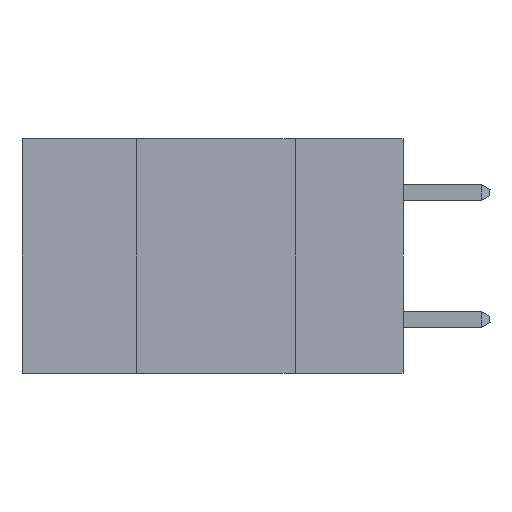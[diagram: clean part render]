
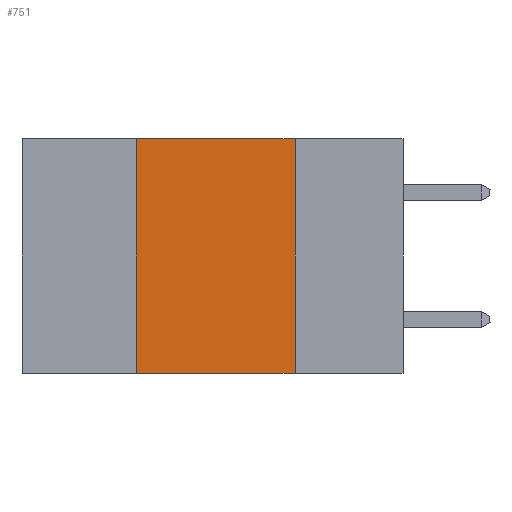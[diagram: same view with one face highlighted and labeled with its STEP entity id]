
A CAD part, left-side view. The second image highlights one B-rep face of the part: STEP entity #751.
In plain terms, the highlighted planar face has unit normal (-1, 0, 0).
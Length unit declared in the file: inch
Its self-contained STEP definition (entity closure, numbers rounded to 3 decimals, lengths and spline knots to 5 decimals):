
#44 = ORIENTED_EDGE ( 'NONE', *, *, #5355, .T. ) ;
#585 = DIRECTION ( 'NONE',  ( 1., 0., 0. ) ) ;
#751 = ADVANCED_FACE ( 'NONE', ( #8405 ), #1571, .F. ) ;
#951 = VERTEX_POINT ( 'NONE', #10991 ) ;
#1030 = AXIS2_PLACEMENT_3D ( 'NONE', #3558, #585, #1523 ) ;
#1355 = CARTESIAN_POINT ( 'NONE',  ( 0., 0.42, 0. ) ) ;
#1523 = DIRECTION ( 'NONE',  ( 0., 0., -1. ) ) ;
#1571 = PLANE ( 'NONE',  #1030 ) ;
#2040 = VECTOR ( 'NONE', #3568, 39.37008 ) ;
#2195 = CARTESIAN_POINT ( 'NONE',  ( 0., 0.17, 0. ) ) ;
#3198 = LINE ( 'NONE', #1355, #9947 ) ;
#3558 = CARTESIAN_POINT ( 'NONE',  ( 0., 0.6, 0. ) ) ;
#3568 = DIRECTION ( 'NONE',  ( 0., -1., 0. ) ) ;
#3680 = CARTESIAN_POINT ( 'NONE',  ( 0., 0.17, 0. ) ) ;
#4013 = LINE ( 'NONE', #2195, #4184 ) ;
#4184 = VECTOR ( 'NONE', #10307, 39.37008 ) ;
#4647 = VERTEX_POINT ( 'NONE', #4947 ) ;
#4910 = CARTESIAN_POINT ( 'NONE',  ( 0., 0.6, 0. ) ) ;
#4947 = CARTESIAN_POINT ( 'NONE',  ( 0., 0.42, -0.37 ) ) ;
#5355 = EDGE_CURVE ( 'NONE', #4647, #7803, #7987, .T. ) ;
#5871 = VECTOR ( 'NONE', #12842, 39.37008 ) ;
#6436 = DIRECTION ( 'NONE',  ( 0., 0., 1. ) ) ;
#7169 = EDGE_LOOP ( 'NONE', ( #7669, #9969, #7737, #44 ) ) ;
#7669 = ORIENTED_EDGE ( 'NONE', *, *, #10270, .F. ) ;
#7737 = ORIENTED_EDGE ( 'NONE', *, *, #11948, .F. ) ;
#7803 = VERTEX_POINT ( 'NONE', #9456 ) ;
#7987 = LINE ( 'NONE', #10544, #2040 ) ;
#8405 = FACE_OUTER_BOUND ( 'NONE', #7169, .T. ) ;
#8692 = LINE ( 'NONE', #4910, #5871 ) ;
#9456 = CARTESIAN_POINT ( 'NONE',  ( 0., 0.17, -0.37 ) ) ;
#9947 = VECTOR ( 'NONE', #6436, 39.37008 ) ;
#9969 = ORIENTED_EDGE ( 'NONE', *, *, #11388, .F. ) ;
#10270 = EDGE_CURVE ( 'NONE', #11546, #7803, #4013, .T. ) ;
#10307 = DIRECTION ( 'NONE',  ( 0., 0., -1. ) ) ;
#10544 = CARTESIAN_POINT ( 'NONE',  ( 0., 0.6, -0.37 ) ) ;
#10991 = CARTESIAN_POINT ( 'NONE',  ( 0., 0.42, 0. ) ) ;
#11388 = EDGE_CURVE ( 'NONE', #951, #11546, #8692, .T. ) ;
#11546 = VERTEX_POINT ( 'NONE', #3680 ) ;
#11948 = EDGE_CURVE ( 'NONE', #4647, #951, #3198, .T. ) ;
#12842 = DIRECTION ( 'NONE',  ( 0., -1., 0. ) ) ;
